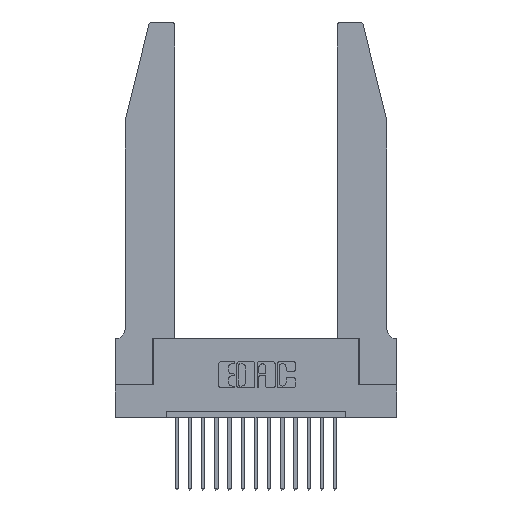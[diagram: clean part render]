
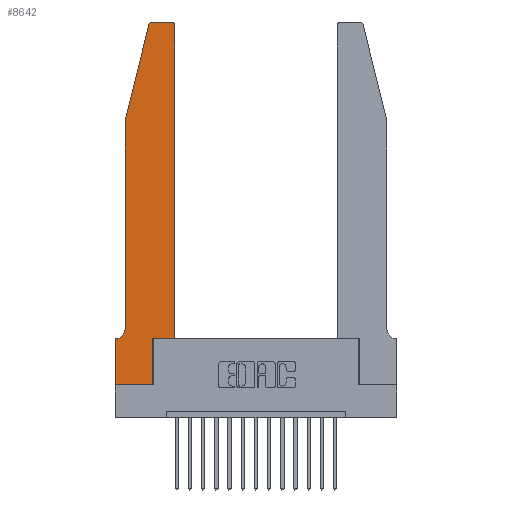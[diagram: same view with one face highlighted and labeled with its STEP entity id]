
A CAD part, top view. The second image highlights one B-rep face of the part: STEP entity #8642.
In plain terms, the highlighted planar face has unit normal (0, 0, 1).
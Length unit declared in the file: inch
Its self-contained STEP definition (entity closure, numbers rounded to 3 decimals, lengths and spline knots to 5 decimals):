
#20 = LINE ( 'NONE', #17984, #4206 ) ;
#207 = DIRECTION ( 'NONE',  ( 0., -1., 0. ) ) ;
#406 = EDGE_CURVE ( 'NONE', #15018, #4752, #2502, .T. ) ;
#407 = VERTEX_POINT ( 'NONE', #847 ) ;
#459 = VECTOR ( 'NONE', #5997, 39.37008 ) ;
#520 = VERTEX_POINT ( 'NONE', #17827 ) ;
#786 = VECTOR ( 'NONE', #2474, 39.37008 ) ;
#800 = CIRCLE ( 'NONE', #2642, 0.03 ) ;
#847 = CARTESIAN_POINT ( 'NONE',  ( 0.284, 2.75, 0.37 ) ) ;
#929 = DIRECTION ( 'NONE',  ( 0., 1., 0. ) ) ;
#1117 = DIRECTION ( 'NONE',  ( -1., 0., 0. ) ) ;
#1218 = CARTESIAN_POINT ( 'NONE',  ( 0.0055, 0.35, 0.37 ) ) ;
#1294 = AXIS2_PLACEMENT_3D ( 'NONE', #10309, #16158, #7601 ) ;
#1533 = CARTESIAN_POINT ( 'NONE',  ( 0.2605, 2.75, 0.37 ) ) ;
#1727 = ORIENTED_EDGE ( 'NONE', *, *, #7050, .T. ) ;
#2474 = DIRECTION ( 'NONE',  ( -0.239, -0.971, 0. ) ) ;
#2502 = LINE ( 'NONE', #13911, #17050 ) ;
#2521 = PLANE ( 'NONE',  #12716 ) ;
#2642 = AXIS2_PLACEMENT_3D ( 'NONE', #4820, #16269, #8968 ) ;
#3014 = LINE ( 'NONE', #17443, #10860 ) ;
#3372 = ORIENTED_EDGE ( 'NONE', *, *, #7779, .T. ) ;
#3946 = VERTEX_POINT ( 'NONE', #11159 ) ;
#4206 = VECTOR ( 'NONE', #13720, 39.37008 ) ;
#4217 = DIRECTION ( 'NONE',  ( -1., 0., 0. ) ) ;
#4505 = ORIENTED_EDGE ( 'NONE', *, *, #13405, .T. ) ;
#4752 = VERTEX_POINT ( 'NONE', #10089 ) ;
#4805 = ORIENTED_EDGE ( 'NONE', *, *, #6924, .T. ) ;
#4820 = CARTESIAN_POINT ( 'NONE',  ( 0.4205, 2.72, 0.37 ) ) ;
#5133 = EDGE_CURVE ( 'NONE', #14872, #15018, #18100, .T. ) ;
#5183 = LINE ( 'NONE', #15151, #15716 ) ;
#5529 = ORIENTED_EDGE ( 'NONE', *, *, #5133, .T. ) ;
#5698 = EDGE_LOOP ( 'NONE', ( #4505, #9453, #3372, #8438, #5529, #9237, #4805, #6799, #12217, #17182, #17165, #1727 ) ) ;
#5840 = VERTEX_POINT ( 'NONE', #16052 ) ;
#5880 = VERTEX_POINT ( 'NONE', #6041 ) ;
#5997 = DIRECTION ( 'NONE',  ( 1., 0., 0. ) ) ;
#6041 = CARTESIAN_POINT ( 'NONE',  ( 0.2865, 0.35, 0.37 ) ) ;
#6129 = CARTESIAN_POINT ( 'NONE',  ( 0., 0., 0.37 ) ) ;
#6391 = DIRECTION ( 'NONE',  ( 0., 1., 0. ) ) ;
#6425 = VERTEX_POINT ( 'NONE', #8161 ) ;
#6434 = CARTESIAN_POINT ( 'NONE',  ( 0.2865, 0., 0.37 ) ) ;
#6530 = VECTOR ( 'NONE', #17048, 39.37008 ) ;
#6531 = CARTESIAN_POINT ( 'NONE',  ( 0.0755, 0.42, 0.37 ) ) ;
#6612 = DIRECTION ( 'NONE',  ( 0., 0., 1. ) ) ;
#6799 = ORIENTED_EDGE ( 'NONE', *, *, #17517, .T. ) ;
#6924 = EDGE_CURVE ( 'NONE', #4752, #3946, #3014, .T. ) ;
#7050 = EDGE_CURVE ( 'NONE', #5840, #15654, #800, .T. ) ;
#7601 = DIRECTION ( 'NONE',  ( 1., 0., 0. ) ) ;
#7779 = EDGE_CURVE ( 'NONE', #13190, #520, #16160, .T. ) ;
#8161 = CARTESIAN_POINT ( 'NONE',  ( 0.4505, 0.35, 0.37 ) ) ;
#8259 = LINE ( 'NONE', #6129, #459 ) ;
#8438 = ORIENTED_EDGE ( 'NONE', *, *, #17428, .T. ) ;
#8642 = ADVANCED_FACE ( 'NONE', ( #17961 ), #2521, .T. ) ;
#8841 = LINE ( 'NONE', #16651, #17348 ) ;
#8968 = DIRECTION ( 'NONE',  ( 1., 0., 0. ) ) ;
#9237 = ORIENTED_EDGE ( 'NONE', *, *, #406, .T. ) ;
#9453 = ORIENTED_EDGE ( 'NONE', *, *, #18267, .T. ) ;
#9700 = DIRECTION ( 'NONE',  ( 1., 0., 0. ) ) ;
#10089 = CARTESIAN_POINT ( 'NONE',  ( 0., 0.35, 0.37 ) ) ;
#10262 = VECTOR ( 'NONE', #207, 39.37008 ) ;
#10309 = CARTESIAN_POINT ( 'NONE',  ( 0.284, 2.72, 0.37 ) ) ;
#10860 = VECTOR ( 'NONE', #15975, 39.37008 ) ;
#11159 = CARTESIAN_POINT ( 'NONE',  ( 0., 0., 0.37 ) ) ;
#11162 = CARTESIAN_POINT ( 'NONE',  ( 0.0755, 2., 0.37 ) ) ;
#12053 = LINE ( 'NONE', #14346, #10262 ) ;
#12119 = EDGE_CURVE ( 'NONE', #17608, #5880, #8841, .T. ) ;
#12217 = ORIENTED_EDGE ( 'NONE', *, *, #12119, .T. ) ;
#12716 = AXIS2_PLACEMENT_3D ( 'NONE', #16840, #6612, #9700 ) ;
#12805 = DIRECTION ( 'NONE',  ( 0., 0., -1. ) ) ;
#13187 = EDGE_CURVE ( 'NONE', #6425, #5840, #5183, .T. ) ;
#13190 = VERTEX_POINT ( 'NONE', #17877 ) ;
#13405 = EDGE_CURVE ( 'NONE', #15654, #407, #17523, .T. ) ;
#13720 = DIRECTION ( 'NONE',  ( 1., 0., 0. ) ) ;
#13911 = CARTESIAN_POINT ( 'NONE',  ( 0.0755, 0.35, 0.37 ) ) ;
#14346 = CARTESIAN_POINT ( 'NONE',  ( 0.0755, 2., 0.37 ) ) ;
#14872 = VERTEX_POINT ( 'NONE', #6531 ) ;
#15018 = VERTEX_POINT ( 'NONE', #1218 ) ;
#15151 = CARTESIAN_POINT ( 'NONE',  ( 0.4505, 0.35, 0.37 ) ) ;
#15654 = VERTEX_POINT ( 'NONE', #15763 ) ;
#15716 = VECTOR ( 'NONE', #6391, 39.37008 ) ;
#15763 = CARTESIAN_POINT ( 'NONE',  ( 0.4205, 2.75, 0.37 ) ) ;
#15976 = EDGE_CURVE ( 'NONE', #5880, #6425, #20, .T. ) ;
#15975 = DIRECTION ( 'NONE',  ( 0., -1., 0. ) ) ;
#16052 = CARTESIAN_POINT ( 'NONE',  ( 0.4505, 2.72, 0.37 ) ) ;
#16158 = DIRECTION ( 'NONE',  ( 0., 0., 1. ) ) ;
#16160 = LINE ( 'NONE', #11162, #786 ) ;
#16269 = DIRECTION ( 'NONE',  ( 0., 0., 1. ) ) ;
#16651 = CARTESIAN_POINT ( 'NONE',  ( 0.2865, 0.35, 0.37 ) ) ;
#16840 = CARTESIAN_POINT ( 'NONE',  ( 0., 0.35, 0.37 ) ) ;
#17048 = DIRECTION ( 'NONE',  ( -1., 0., 0. ) ) ;
#17050 = VECTOR ( 'NONE', #1117, 39.37008 ) ;
#17165 = ORIENTED_EDGE ( 'NONE', *, *, #13187, .T. ) ;
#17182 = ORIENTED_EDGE ( 'NONE', *, *, #15976, .T. ) ;
#17348 = VECTOR ( 'NONE', #929, 39.37008 ) ;
#17428 = EDGE_CURVE ( 'NONE', #520, #14872, #12053, .T. ) ;
#17443 = CARTESIAN_POINT ( 'NONE',  ( 0., 0., 0.37 ) ) ;
#17485 = AXIS2_PLACEMENT_3D ( 'NONE', #18382, #12805, #4217 ) ;
#17517 = EDGE_CURVE ( 'NONE', #3946, #17608, #8259, .T. ) ;
#17523 = LINE ( 'NONE', #1533, #6530 ) ;
#17608 = VERTEX_POINT ( 'NONE', #6434 ) ;
#17615 = CIRCLE ( 'NONE', #1294, 0.03 ) ;
#17827 = CARTESIAN_POINT ( 'NONE',  ( 0.0755, 2., 0.37 ) ) ;
#17877 = CARTESIAN_POINT ( 'NONE',  ( 0.25487, 2.72718, 0.37 ) ) ;
#17961 = FACE_OUTER_BOUND ( 'NONE', #5698, .T. ) ;
#17984 = CARTESIAN_POINT ( 'NONE',  ( 0.4505, 0.35, 0.37 ) ) ;
#18100 = CIRCLE ( 'NONE', #17485, 0.07 ) ;
#18267 = EDGE_CURVE ( 'NONE', #407, #13190, #17615, .T. ) ;
#18382 = CARTESIAN_POINT ( 'NONE',  ( 0.0055, 0.42, 0.37 ) ) ;
